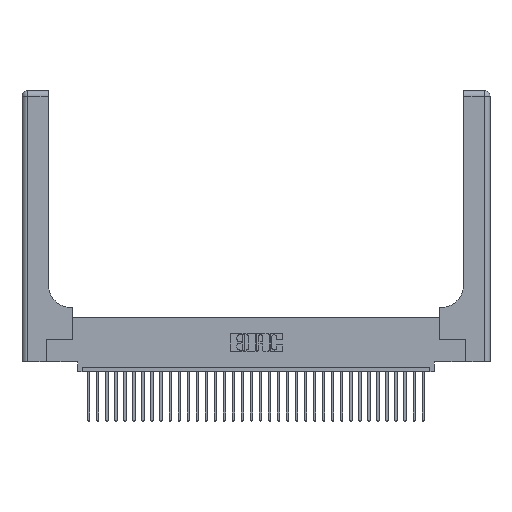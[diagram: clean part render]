
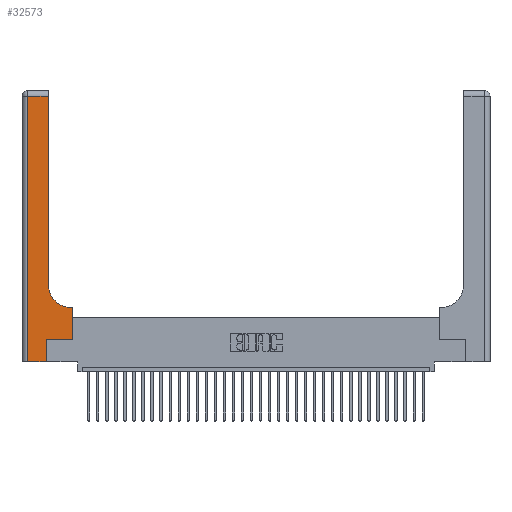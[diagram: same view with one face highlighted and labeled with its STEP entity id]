
A CAD part, top view. The second image highlights one B-rep face of the part: STEP entity #32573.
In plain terms, the highlighted planar face has unit normal (0, 0, 1).
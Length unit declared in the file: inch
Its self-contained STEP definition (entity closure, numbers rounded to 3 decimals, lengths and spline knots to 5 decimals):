
#261 = DIRECTION ( 'NONE',  ( 0., 1., 0. ) ) ;
#797 = CARTESIAN_POINT ( 'NONE',  ( 0.5415, 0.6, 0.37 ) ) ;
#2353 = DIRECTION ( 'NONE',  ( 0., 0., -1. ) ) ;
#2377 = VECTOR ( 'NONE', #14169, 39.37008 ) ;
#2477 = CARTESIAN_POINT ( 'NONE',  ( 0., 2.94, 0.37 ) ) ;
#2813 = EDGE_CURVE ( 'NONE', #15145, #14686, #29455, .T. ) ;
#3087 = VERTEX_POINT ( 'NONE', #3865 ) ;
#3483 = LINE ( 'NONE', #2477, #6838 ) ;
#3865 = CARTESIAN_POINT ( 'NONE',  ( 0.06, 2.94, 0.37 ) ) ;
#3901 = AXIS2_PLACEMENT_3D ( 'NONE', #29384, #5736, #32080 ) ;
#4811 = ORIENTED_EDGE ( 'NONE', *, *, #5236, .T. ) ;
#4914 = ORIENTED_EDGE ( 'NONE', *, *, #28106, .T. ) ;
#5236 = EDGE_CURVE ( 'NONE', #7489, #31074, #15955, .T. ) ;
#5471 = AXIS2_PLACEMENT_3D ( 'NONE', #7221, #2353, #20943 ) ;
#5736 = DIRECTION ( 'NONE',  ( 0., 0., -1. ) ) ;
#6436 = CARTESIAN_POINT ( 'NONE',  ( 0.5585, 0.6, 0.37 ) ) ;
#6803 = VERTEX_POINT ( 'NONE', #18233 ) ;
#6838 = VECTOR ( 'NONE', #22472, 39.37008 ) ;
#6868 = EDGE_LOOP ( 'NONE', ( #16411, #24044, #4914, #4811, #26825, #24916, #14068, #26663, #26695 ) ) ;
#7221 = CARTESIAN_POINT ( 'NONE',  ( 0.5415, 0.85, 0.37 ) ) ;
#7489 = VERTEX_POINT ( 'NONE', #12601 ) ;
#7531 = CIRCLE ( 'NONE', #5471, 0.25 ) ;
#7979 = CARTESIAN_POINT ( 'NONE',  ( 0., 0., 0.37 ) ) ;
#8050 = LINE ( 'NONE', #9366, #28440 ) ;
#8813 = DIRECTION ( 'NONE',  ( -1., 0., 0. ) ) ;
#9366 = CARTESIAN_POINT ( 'NONE',  ( 0.2915, 3., 0.37 ) ) ;
#9400 = EDGE_CURVE ( 'NONE', #6803, #19862, #8050, .T. ) ;
#9586 = VECTOR ( 'NONE', #8813, 39.37008 ) ;
#9831 = CARTESIAN_POINT ( 'NONE',  ( 0.2915, 2.94, 0.37 ) ) ;
#10423 = EDGE_CURVE ( 'NONE', #31074, #20061, #10924, .T. ) ;
#10725 = CARTESIAN_POINT ( 'NONE',  ( 0.5585, 0.25, 0.37 ) ) ;
#10924 = LINE ( 'NONE', #31408, #31316 ) ;
#11778 = DIRECTION ( 'NONE',  ( 0., 1., 0. ) ) ;
#11841 = CARTESIAN_POINT ( 'NONE',  ( 0.06, 3., 0.37 ) ) ;
#12601 = CARTESIAN_POINT ( 'NONE',  ( 0.06, 0., 0.37 ) ) ;
#13052 = CARTESIAN_POINT ( 'NONE',  ( 0.269, 0.25, 0.37 ) ) ;
#13476 = PLANE ( 'NONE',  #3901 ) ;
#14068 = ORIENTED_EDGE ( 'NONE', *, *, #2813, .T. ) ;
#14169 = DIRECTION ( 'NONE',  ( 0., -1., 0. ) ) ;
#14686 = VERTEX_POINT ( 'NONE', #6436 ) ;
#15145 = VERTEX_POINT ( 'NONE', #10725 ) ;
#15262 = EDGE_CURVE ( 'NONE', #14686, #15581, #24087, .T. ) ;
#15333 = VECTOR ( 'NONE', #261, 39.37008 ) ;
#15403 = FACE_OUTER_BOUND ( 'NONE', #6868, .T. ) ;
#15581 = VERTEX_POINT ( 'NONE', #797 ) ;
#15955 = LINE ( 'NONE', #7979, #20540 ) ;
#16052 = LINE ( 'NONE', #11841, #2377 ) ;
#16411 = ORIENTED_EDGE ( 'NONE', *, *, #9400, .T. ) ;
#17091 = DIRECTION ( 'NONE',  ( 1., 0., 0. ) ) ;
#18233 = CARTESIAN_POINT ( 'NONE',  ( 0.2915, 0.85, 0.37 ) ) ;
#18640 = EDGE_CURVE ( 'NONE', #19862, #3087, #3483, .T. ) ;
#19862 = VERTEX_POINT ( 'NONE', #9831 ) ;
#20061 = VERTEX_POINT ( 'NONE', #13052 ) ;
#20540 = VECTOR ( 'NONE', #17091, 39.37008 ) ;
#20943 = DIRECTION ( 'NONE',  ( 1., 0., 0. ) ) ;
#21138 = DIRECTION ( 'NONE',  ( 0., 1., 0. ) ) ;
#22057 = CARTESIAN_POINT ( 'NONE',  ( 0.2915, 0.6, 0.37 ) ) ;
#22472 = DIRECTION ( 'NONE',  ( -1., 0., 0. ) ) ;
#23794 = EDGE_CURVE ( 'NONE', #20061, #15145, #30098, .T. ) ;
#24044 = ORIENTED_EDGE ( 'NONE', *, *, #18640, .T. ) ;
#24086 = DIRECTION ( 'NONE',  ( 1., 0., 0. ) ) ;
#24087 = LINE ( 'NONE', #22057, #9586 ) ;
#24472 = CARTESIAN_POINT ( 'NONE',  ( 0.5585, 0.25, 0.37 ) ) ;
#24916 = ORIENTED_EDGE ( 'NONE', *, *, #23794, .T. ) ;
#26663 = ORIENTED_EDGE ( 'NONE', *, *, #15262, .T. ) ;
#26695 = ORIENTED_EDGE ( 'NONE', *, *, #33624, .T. ) ;
#26825 = ORIENTED_EDGE ( 'NONE', *, *, #10423, .T. ) ;
#28106 = EDGE_CURVE ( 'NONE', #3087, #7489, #16052, .T. ) ;
#28440 = VECTOR ( 'NONE', #11778, 39.37008 ) ;
#29384 = CARTESIAN_POINT ( 'NONE',  ( 0., 3., 0.37 ) ) ;
#29455 = LINE ( 'NONE', #24472, #15333 ) ;
#29928 = CARTESIAN_POINT ( 'NONE',  ( 0.269, 0.25, 0.37 ) ) ;
#30098 = LINE ( 'NONE', #29928, #31821 ) ;
#31074 = VERTEX_POINT ( 'NONE', #31626 ) ;
#31316 = VECTOR ( 'NONE', #21138, 39.37008 ) ;
#31408 = CARTESIAN_POINT ( 'NONE',  ( 0.269, 0., 0.37 ) ) ;
#31626 = CARTESIAN_POINT ( 'NONE',  ( 0.269, 0., 0.37 ) ) ;
#31821 = VECTOR ( 'NONE', #24086, 39.37008 ) ;
#32080 = DIRECTION ( 'NONE',  ( -1., 0., 0. ) ) ;
#32573 = ADVANCED_FACE ( 'NONE', ( #15403 ), #13476, .F. ) ;
#33624 = EDGE_CURVE ( 'NONE', #15581, #6803, #7531, .T. ) ;
